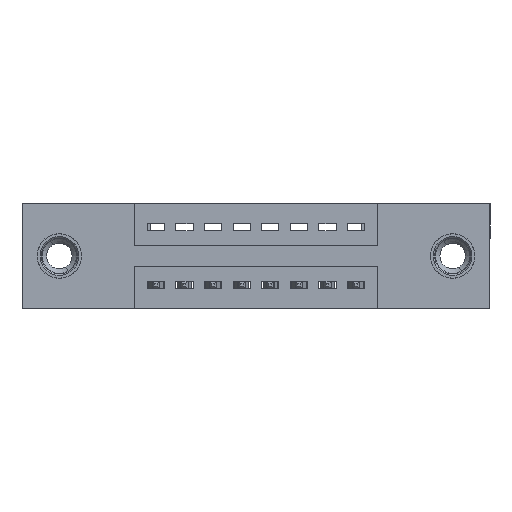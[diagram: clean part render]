
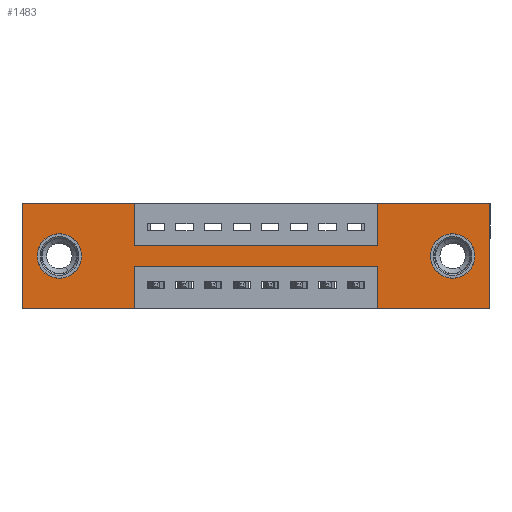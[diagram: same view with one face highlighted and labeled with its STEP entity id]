
A CAD part, front view. The second image highlights one B-rep face of the part: STEP entity #1483.
In plain terms, the highlighted planar face has unit normal (0, -1, 0).
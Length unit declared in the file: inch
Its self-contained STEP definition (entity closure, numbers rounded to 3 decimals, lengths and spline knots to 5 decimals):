
#84 = ORIENTED_EDGE ( 'NONE', *, *, #7727, .F. ) ;
#139 = LINE ( 'NONE', #3155, #1854 ) ;
#193 = DIRECTION ( 'NONE',  ( 0., 0., 1. ) ) ;
#231 = EDGE_CURVE ( 'NONE', #294, #5429, #10033, .T. ) ;
#247 = ORIENTED_EDGE ( 'NONE', *, *, #5558, .F. ) ;
#294 = VERTEX_POINT ( 'NONE', #3681 ) ;
#341 = PLANE ( 'NONE',  #6576 ) ;
#470 = VERTEX_POINT ( 'NONE', #3360 ) ;
#492 = CARTESIAN_POINT ( 'NONE',  ( 1.635, 0., 0. ) ) ;
#552 = VECTOR ( 'NONE', #5226, 39.37008 ) ;
#715 = ORIENTED_EDGE ( 'NONE', *, *, #11618, .T. ) ;
#855 = CARTESIAN_POINT ( 'NONE',  ( 0.3925, 0., -0.22 ) ) ;
#985 = ORIENTED_EDGE ( 'NONE', *, *, #2270, .T. ) ;
#1014 = VERTEX_POINT ( 'NONE', #11260 ) ;
#1146 = CARTESIAN_POINT ( 'NONE',  ( 1.2425, 0., -0.22 ) ) ;
#1176 = LINE ( 'NONE', #2265, #552 ) ;
#1253 = CIRCLE ( 'NONE', #5135, 0.078 ) ;
#1393 = VERTEX_POINT ( 'NONE', #8900 ) ;
#1483 = ADVANCED_FACE ( 'NONE', ( #7688, #4268, #11834 ), #341, .T. ) ;
#1533 = CARTESIAN_POINT ( 'NONE',  ( 1.2425, 0., 0. ) ) ;
#1833 = ORIENTED_EDGE ( 'NONE', *, *, #5437, .T. ) ;
#1844 = LINE ( 'NONE', #9220, #12640 ) ;
#1854 = VECTOR ( 'NONE', #193, 39.37008 ) ;
#1911 = ORIENTED_EDGE ( 'NONE', *, *, #12607, .F. ) ;
#1937 = LINE ( 'NONE', #3210, #5649 ) ;
#2002 = VERTEX_POINT ( 'NONE', #2103 ) ;
#2103 = CARTESIAN_POINT ( 'NONE',  ( 0.3925, 0., -0.15 ) ) ;
#2139 = CARTESIAN_POINT ( 'NONE',  ( 0., 0., 0. ) ) ;
#2144 = DIRECTION ( 'NONE',  ( 0., 1., 0. ) ) ;
#2265 = CARTESIAN_POINT ( 'NONE',  ( 0., 0., 0. ) ) ;
#2270 = EDGE_CURVE ( 'NONE', #11613, #2799, #11954, .T. ) ;
#2336 = VECTOR ( 'NONE', #9060, 39.37008 ) ;
#2380 = DIRECTION ( 'NONE',  ( 0., 0., -1. ) ) ;
#2669 = ORIENTED_EDGE ( 'NONE', *, *, #7084, .F. ) ;
#2799 = VERTEX_POINT ( 'NONE', #2964 ) ;
#2923 = EDGE_CURVE ( 'NONE', #470, #8393, #1937, .T. ) ;
#2964 = CARTESIAN_POINT ( 'NONE',  ( 1.505, 0., -0.263 ) ) ;
#3155 = CARTESIAN_POINT ( 'NONE',  ( 1.2425, 0., -0.37 ) ) ;
#3210 = CARTESIAN_POINT ( 'NONE',  ( 0., 0., -0.37 ) ) ;
#3222 = CARTESIAN_POINT ( 'NONE',  ( 0.3925, 0., 0. ) ) ;
#3229 = DIRECTION ( 'NONE',  ( 0., -1., 0. ) ) ;
#3319 = CARTESIAN_POINT ( 'NONE',  ( 0., 0., -0.37 ) ) ;
#3329 = EDGE_LOOP ( 'NONE', ( #985, #4938 ) ) ;
#3360 = CARTESIAN_POINT ( 'NONE',  ( 1.635, 0., -0.37 ) ) ;
#3498 = LINE ( 'NONE', #6514, #8281 ) ;
#3569 = VECTOR ( 'NONE', #6740, 39.37008 ) ;
#3681 = CARTESIAN_POINT ( 'NONE',  ( 0.3925, 0., -0.22 ) ) ;
#3713 = CARTESIAN_POINT ( 'NONE',  ( 0.3925, 0., 0. ) ) ;
#3875 = ORIENTED_EDGE ( 'NONE', *, *, #8534, .F. ) ;
#4268 = FACE_BOUND ( 'NONE', #12300, .T. ) ;
#4270 = AXIS2_PLACEMENT_3D ( 'NONE', #9994, #2144, #11921 ) ;
#4640 = ORIENTED_EDGE ( 'NONE', *, *, #5213, .F. ) ;
#4723 = VECTOR ( 'NONE', #7123, 39.37008 ) ;
#4938 = ORIENTED_EDGE ( 'NONE', *, *, #11444, .T. ) ;
#4941 = VERTEX_POINT ( 'NONE', #10031 ) ;
#4956 = EDGE_LOOP ( 'NONE', ( #8970, #4640, #1911, #7938, #2669, #84, #7395, #247, #9295, #3875, #8413, #10177 ) ) ;
#5075 = EDGE_CURVE ( 'NONE', #1014, #8844, #6794, .T. ) ;
#5135 = AXIS2_PLACEMENT_3D ( 'NONE', #8606, #6605, #10540 ) ;
#5176 = AXIS2_PLACEMENT_3D ( 'NONE', #5873, #9758, #5920 ) ;
#5213 = EDGE_CURVE ( 'NONE', #10579, #294, #9891, .T. ) ;
#5226 = DIRECTION ( 'NONE',  ( 0., 0., 1. ) ) ;
#5317 = AXIS2_PLACEMENT_3D ( 'NONE', #5828, #11819, #9756 ) ;
#5330 = CARTESIAN_POINT ( 'NONE',  ( 0.13, 0., -0.263 ) ) ;
#5429 = VERTEX_POINT ( 'NONE', #5576 ) ;
#5437 = EDGE_CURVE ( 'NONE', #6838, #4941, #1253, .T. ) ;
#5504 = LINE ( 'NONE', #2139, #4723 ) ;
#5558 = EDGE_CURVE ( 'NONE', #2002, #1014, #9423, .T. ) ;
#5576 = CARTESIAN_POINT ( 'NONE',  ( 0.3925, 0., -0.37 ) ) ;
#5595 = VERTEX_POINT ( 'NONE', #6407 ) ;
#5649 = VECTOR ( 'NONE', #10039, 39.37008 ) ;
#5745 = VERTEX_POINT ( 'NONE', #10601 ) ;
#5828 = CARTESIAN_POINT ( 'NONE',  ( 0.13, 0., -0.185 ) ) ;
#5873 = CARTESIAN_POINT ( 'NONE',  ( 1.505, 0., -0.185 ) ) ;
#5920 = DIRECTION ( 'NONE',  ( 0., 0., -1. ) ) ;
#6303 = DIRECTION ( 'NONE',  ( 0., 0., -1. ) ) ;
#6407 = CARTESIAN_POINT ( 'NONE',  ( 0., 0., -0.37 ) ) ;
#6454 = CARTESIAN_POINT ( 'NONE',  ( 0.3925, 0., -0.15 ) ) ;
#6514 = CARTESIAN_POINT ( 'NONE',  ( 0., 0., 0. ) ) ;
#6576 = AXIS2_PLACEMENT_3D ( 'NONE', #3319, #3229, #2380 ) ;
#6605 = DIRECTION ( 'NONE',  ( 0., 1., 0. ) ) ;
#6740 = DIRECTION ( 'NONE',  ( -1., 0., 0. ) ) ;
#6790 = EDGE_CURVE ( 'NONE', #5429, #5595, #1844, .T. ) ;
#6794 = LINE ( 'NONE', #1533, #2336 ) ;
#6838 = VERTEX_POINT ( 'NONE', #5330 ) ;
#6936 = CARTESIAN_POINT ( 'NONE',  ( 1.2425, 0., -0.37 ) ) ;
#7084 = EDGE_CURVE ( 'NONE', #1393, #470, #9234, .T. ) ;
#7123 = DIRECTION ( 'NONE',  ( 1., 0., 0. ) ) ;
#7211 = EDGE_CURVE ( 'NONE', #5595, #5745, #1176, .T. ) ;
#7235 = DIRECTION ( 'NONE',  ( 0., 0., -1. ) ) ;
#7388 = DIRECTION ( 'NONE',  ( 0., 0., -1. ) ) ;
#7395 = ORIENTED_EDGE ( 'NONE', *, *, #5075, .F. ) ;
#7688 = FACE_BOUND ( 'NONE', #3329, .T. ) ;
#7727 = EDGE_CURVE ( 'NONE', #8844, #1393, #3498, .T. ) ;
#7735 = VECTOR ( 'NONE', #11408, 39.37008 ) ;
#7938 = ORIENTED_EDGE ( 'NONE', *, *, #2923, .F. ) ;
#8033 = LINE ( 'NONE', #3222, #12496 ) ;
#8281 = VECTOR ( 'NONE', #12343, 39.37008 ) ;
#8393 = VERTEX_POINT ( 'NONE', #6936 ) ;
#8413 = ORIENTED_EDGE ( 'NONE', *, *, #7211, .F. ) ;
#8534 = EDGE_CURVE ( 'NONE', #5745, #10621, #5504, .T. ) ;
#8606 = CARTESIAN_POINT ( 'NONE',  ( 0.13, 0., -0.185 ) ) ;
#8844 = VERTEX_POINT ( 'NONE', #11325 ) ;
#8900 = CARTESIAN_POINT ( 'NONE',  ( 1.635, 0., 0. ) ) ;
#8970 = ORIENTED_EDGE ( 'NONE', *, *, #231, .F. ) ;
#9060 = DIRECTION ( 'NONE',  ( 0., 0., 1. ) ) ;
#9220 = CARTESIAN_POINT ( 'NONE',  ( 0., 0., -0.37 ) ) ;
#9234 = LINE ( 'NONE', #492, #9394 ) ;
#9278 = CIRCLE ( 'NONE', #4270, 0.078 ) ;
#9295 = ORIENTED_EDGE ( 'NONE', *, *, #11643, .F. ) ;
#9311 = DIRECTION ( 'NONE',  ( -1., 0., 0. ) ) ;
#9394 = VECTOR ( 'NONE', #7388, 39.37008 ) ;
#9423 = LINE ( 'NONE', #6454, #7735 ) ;
#9756 = DIRECTION ( 'NONE',  ( 0., 0., 1. ) ) ;
#9758 = DIRECTION ( 'NONE',  ( 0., 1., 0. ) ) ;
#9891 = LINE ( 'NONE', #855, #3569 ) ;
#9994 = CARTESIAN_POINT ( 'NONE',  ( 1.505, 0., -0.185 ) ) ;
#10031 = CARTESIAN_POINT ( 'NONE',  ( 0.13, 0., -0.107 ) ) ;
#10033 = LINE ( 'NONE', #12218, #10196 ) ;
#10039 = DIRECTION ( 'NONE',  ( -1., 0., 0. ) ) ;
#10177 = ORIENTED_EDGE ( 'NONE', *, *, #6790, .F. ) ;
#10196 = VECTOR ( 'NONE', #6303, 39.37008 ) ;
#10540 = DIRECTION ( 'NONE',  ( 0., 0., 1. ) ) ;
#10579 = VERTEX_POINT ( 'NONE', #1146 ) ;
#10601 = CARTESIAN_POINT ( 'NONE',  ( 0., 0., 0. ) ) ;
#10621 = VERTEX_POINT ( 'NONE', #3713 ) ;
#11260 = CARTESIAN_POINT ( 'NONE',  ( 1.2425, 0., -0.15 ) ) ;
#11325 = CARTESIAN_POINT ( 'NONE',  ( 1.2425, 0., 0. ) ) ;
#11408 = DIRECTION ( 'NONE',  ( 1., 0., 0. ) ) ;
#11444 = EDGE_CURVE ( 'NONE', #2799, #11613, #9278, .T. ) ;
#11613 = VERTEX_POINT ( 'NONE', #12736 ) ;
#11618 = EDGE_CURVE ( 'NONE', #4941, #6838, #11743, .T. ) ;
#11643 = EDGE_CURVE ( 'NONE', #10621, #2002, #8033, .T. ) ;
#11743 = CIRCLE ( 'NONE', #5317, 0.078 ) ;
#11819 = DIRECTION ( 'NONE',  ( 0., 1., 0. ) ) ;
#11834 = FACE_OUTER_BOUND ( 'NONE', #4956, .T. ) ;
#11921 = DIRECTION ( 'NONE',  ( 0., 0., -1. ) ) ;
#11954 = CIRCLE ( 'NONE', #5176, 0.078 ) ;
#12218 = CARTESIAN_POINT ( 'NONE',  ( 0.3925, 0., -0.37 ) ) ;
#12300 = EDGE_LOOP ( 'NONE', ( #715, #1833 ) ) ;
#12343 = DIRECTION ( 'NONE',  ( 1., 0., 0. ) ) ;
#12496 = VECTOR ( 'NONE', #7235, 39.37008 ) ;
#12607 = EDGE_CURVE ( 'NONE', #8393, #10579, #139, .T. ) ;
#12640 = VECTOR ( 'NONE', #9311, 39.37008 ) ;
#12736 = CARTESIAN_POINT ( 'NONE',  ( 1.505, 0., -0.107 ) ) ;
